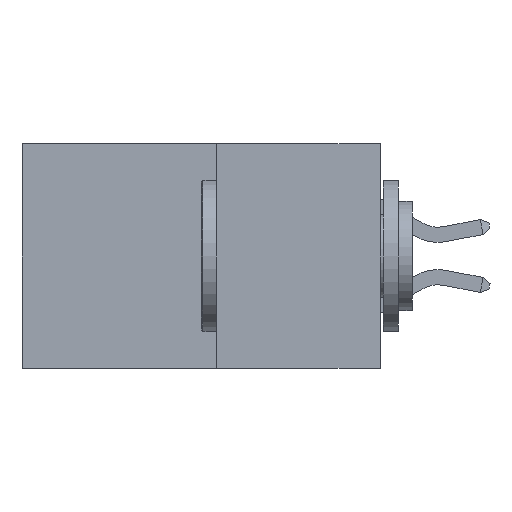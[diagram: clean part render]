
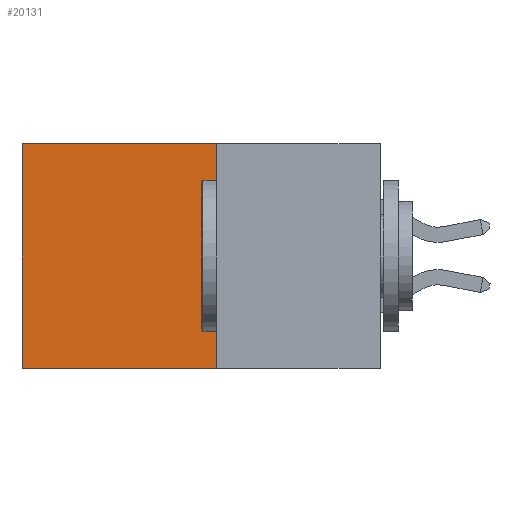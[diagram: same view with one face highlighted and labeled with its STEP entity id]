
A CAD part, left-side view. The second image highlights one B-rep face of the part: STEP entity #20131.
In plain terms, the highlighted planar face has unit normal (-1, 0, 0).
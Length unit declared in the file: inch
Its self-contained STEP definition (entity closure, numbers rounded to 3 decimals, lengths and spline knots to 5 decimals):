
#1268 = VECTOR ( 'NONE', #17567, 39.37008 ) ;
#1304 = CARTESIAN_POINT ( 'NONE',  ( 0.277, 0.27, 0. ) ) ;
#1439 = LINE ( 'NONE', #1304, #9823 ) ;
#1839 = LINE ( 'NONE', #3445, #1268 ) ;
#2884 = EDGE_LOOP ( 'NONE', ( #18152, #4646, #20554, #20578 ) ) ;
#3326 = AXIS2_PLACEMENT_3D ( 'NONE', #4747, #8345, #20549 ) ;
#3445 = CARTESIAN_POINT ( 'NONE',  ( 0.277, 0.27, -0.37 ) ) ;
#4646 = ORIENTED_EDGE ( 'NONE', *, *, #9719, .F. ) ;
#4747 = CARTESIAN_POINT ( 'NONE',  ( 0.277, 0.27, -0.37 ) ) ;
#6547 = PLANE ( 'NONE',  #3326 ) ;
#6918 = VECTOR ( 'NONE', #9559, 39.37008 ) ;
#7228 = DIRECTION ( 'NONE',  ( 0., 0., -1. ) ) ;
#7397 = EDGE_CURVE ( 'NONE', #12779, #10319, #1839, .T. ) ;
#7475 = VERTEX_POINT ( 'NONE', #8993 ) ;
#8345 = DIRECTION ( 'NONE',  ( 1., 0., 0. ) ) ;
#8993 = CARTESIAN_POINT ( 'NONE',  ( 0.277, 0.59, 0. ) ) ;
#9371 = VECTOR ( 'NONE', #7228, 39.37008 ) ;
#9559 = DIRECTION ( 'NONE',  ( 0., 1., 0. ) ) ;
#9676 = CARTESIAN_POINT ( 'NONE',  ( 0.277, 0.59, -0.37 ) ) ;
#9719 = EDGE_CURVE ( 'NONE', #10319, #13094, #20322, .T. ) ;
#9823 = VECTOR ( 'NONE', #11958, 39.37008 ) ;
#10319 = VERTEX_POINT ( 'NONE', #14428 ) ;
#10419 = CARTESIAN_POINT ( 'NONE',  ( 0.277, 0.27, 0. ) ) ;
#11958 = DIRECTION ( 'NONE',  ( 0., 1., 0. ) ) ;
#12683 = EDGE_CURVE ( 'NONE', #12779, #7475, #1439, .T. ) ;
#12779 = VERTEX_POINT ( 'NONE', #10419 ) ;
#13094 = VERTEX_POINT ( 'NONE', #9676 ) ;
#13431 = FACE_OUTER_BOUND ( 'NONE', #2884, .T. ) ;
#14022 = LINE ( 'NONE', #17748, #9371 ) ;
#14428 = CARTESIAN_POINT ( 'NONE',  ( 0.277, 0.27, -0.37 ) ) ;
#17567 = DIRECTION ( 'NONE',  ( 0., 0., -1. ) ) ;
#17748 = CARTESIAN_POINT ( 'NONE',  ( 0.277, 0.59, -0.37 ) ) ;
#18152 = ORIENTED_EDGE ( 'NONE', *, *, #18702, .T. ) ;
#18702 = EDGE_CURVE ( 'NONE', #7475, #13094, #14022, .T. ) ;
#19996 = CARTESIAN_POINT ( 'NONE',  ( 0.277, 0.27, -0.37 ) ) ;
#20131 = ADVANCED_FACE ( 'NONE', ( #13431 ), #6547, .F. ) ;
#20322 = LINE ( 'NONE', #19996, #6918 ) ;
#20549 = DIRECTION ( 'NONE',  ( 0., 0., -1. ) ) ;
#20554 = ORIENTED_EDGE ( 'NONE', *, *, #7397, .F. ) ;
#20578 = ORIENTED_EDGE ( 'NONE', *, *, #12683, .T. ) ;
